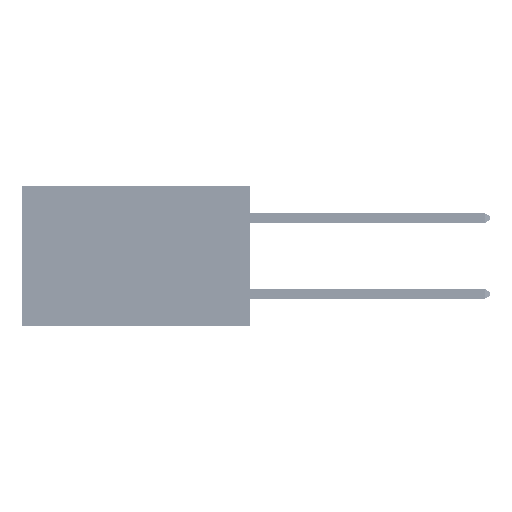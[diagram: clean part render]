
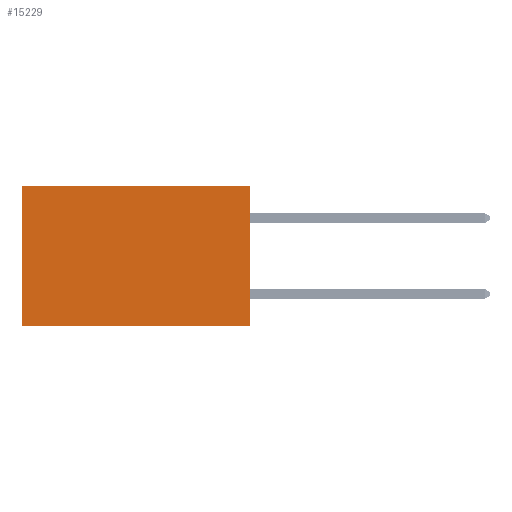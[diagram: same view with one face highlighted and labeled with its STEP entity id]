
A CAD part, left-side view. The second image highlights one B-rep face of the part: STEP entity #15229.
In plain terms, the highlighted planar face has unit normal (-1, 0, 0).
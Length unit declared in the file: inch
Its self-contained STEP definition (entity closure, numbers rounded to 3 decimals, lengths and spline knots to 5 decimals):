
#2370 = LINE ( 'NONE', #11356, #33474 ) ;
#3502 = CARTESIAN_POINT ( 'NONE',  ( 0.2875, 0., 0. ) ) ;
#3678 = DIRECTION ( 'NONE',  ( 0., 0., -1. ) ) ;
#7343 = ORIENTED_EDGE ( 'NONE', *, *, #33287, .F. ) ;
#8142 = EDGE_LOOP ( 'NONE', ( #8201, #41384, #7343, #26998 ) ) ;
#8201 = ORIENTED_EDGE ( 'NONE', *, *, #13034, .T. ) ;
#10297 = CARTESIAN_POINT ( 'NONE',  ( 0.2875, 0., -0.37 ) ) ;
#11356 = CARTESIAN_POINT ( 'NONE',  ( 0.2875, 0.6, 0. ) ) ;
#13034 = EDGE_CURVE ( 'NONE', #43588, #28043, #2370, .T. ) ;
#14410 = DIRECTION ( 'NONE',  ( 0., 1., 0. ) ) ;
#15229 = ADVANCED_FACE ( 'NONE', ( #39496 ), #40471, .F. ) ;
#15314 = CARTESIAN_POINT ( 'NONE',  ( 0.2875, 0.6, 0. ) ) ;
#16934 = VECTOR ( 'NONE', #49982, 39.37008 ) ;
#20813 = EDGE_CURVE ( 'NONE', #37503, #28043, #31410, .T. ) ;
#22028 = CARTESIAN_POINT ( 'NONE',  ( 0.2875, 0., 0. ) ) ;
#24188 = AXIS2_PLACEMENT_3D ( 'NONE', #36472, #48300, #44441 ) ;
#24207 = CARTESIAN_POINT ( 'NONE',  ( 0.2875, 0., 0. ) ) ;
#24566 = LINE ( 'NONE', #22028, #16934 ) ;
#26998 = ORIENTED_EDGE ( 'NONE', *, *, #49968, .T. ) ;
#28043 = VERTEX_POINT ( 'NONE', #31226 ) ;
#31226 = CARTESIAN_POINT ( 'NONE',  ( 0.2875, 0.6, -0.37 ) ) ;
#31410 = LINE ( 'NONE', #10297, #40802 ) ;
#33287 = EDGE_CURVE ( 'NONE', #48970, #37503, #47475, .T. ) ;
#33474 = VECTOR ( 'NONE', #35507, 39.37008 ) ;
#35507 = DIRECTION ( 'NONE',  ( 0., 0., -1. ) ) ;
#36472 = CARTESIAN_POINT ( 'NONE',  ( 0.2875, 0., 0. ) ) ;
#36891 = VECTOR ( 'NONE', #3678, 39.37008 ) ;
#37024 = CARTESIAN_POINT ( 'NONE',  ( 0.2875, 0., -0.37 ) ) ;
#37503 = VERTEX_POINT ( 'NONE', #37024 ) ;
#39496 = FACE_OUTER_BOUND ( 'NONE', #8142, .T. ) ;
#40471 = PLANE ( 'NONE',  #24188 ) ;
#40802 = VECTOR ( 'NONE', #14410, 39.37008 ) ;
#41384 = ORIENTED_EDGE ( 'NONE', *, *, #20813, .F. ) ;
#43588 = VERTEX_POINT ( 'NONE', #15314 ) ;
#44441 = DIRECTION ( 'NONE',  ( 0., 0., -1. ) ) ;
#47475 = LINE ( 'NONE', #3502, #36891 ) ;
#48300 = DIRECTION ( 'NONE',  ( 1., 0., 0. ) ) ;
#48970 = VERTEX_POINT ( 'NONE', #24207 ) ;
#49968 = EDGE_CURVE ( 'NONE', #48970, #43588, #24566, .T. ) ;
#49982 = DIRECTION ( 'NONE',  ( 0., 1., 0. ) ) ;
